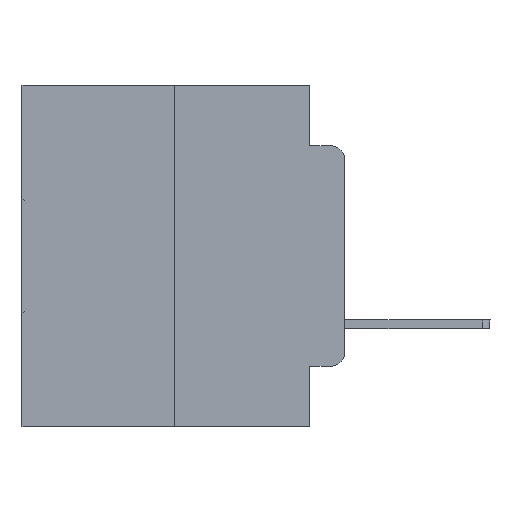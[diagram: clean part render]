
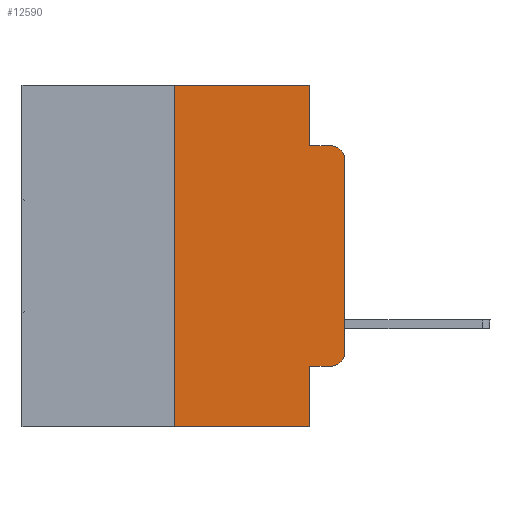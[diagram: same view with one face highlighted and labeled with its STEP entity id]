
A CAD part, left-side view. The second image highlights one B-rep face of the part: STEP entity #12590.
In plain terms, the highlighted planar face has unit normal (-1, 0, 0).
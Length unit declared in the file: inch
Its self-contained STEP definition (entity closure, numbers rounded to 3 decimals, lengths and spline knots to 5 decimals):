
#185 = DIRECTION ( 'NONE',  ( 0., -1., 0. ) ) ;
#440 = DIRECTION ( 'NONE',  ( 0., 0., -1. ) ) ;
#612 = CARTESIAN_POINT ( 'NONE',  ( 0., 0.051, -0.4115 ) ) ;
#1072 = VERTEX_POINT ( 'NONE', #17011 ) ;
#1355 = DIRECTION ( 'NONE',  ( 0., 0., 1. ) ) ;
#2196 = ORIENTED_EDGE ( 'NONE', *, *, #22453, .T. ) ;
#3520 = EDGE_CURVE ( 'NONE', #7182, #22280, #6328, .T. ) ;
#4024 = VECTOR ( 'NONE', #1355, 39.37008 ) ;
#4869 = VECTOR ( 'NONE', #11250, 39.37008 ) ;
#4883 = DIRECTION ( 'NONE',  ( 0., -1., 0. ) ) ;
#5035 = LINE ( 'NONE', #18570, #28274 ) ;
#5258 = LINE ( 'NONE', #19544, #15600 ) ;
#5340 = CARTESIAN_POINT ( 'NONE',  ( 0., 0.473, 0. ) ) ;
#5604 = CARTESIAN_POINT ( 'NONE',  ( 0., 0., 0. ) ) ;
#5632 = EDGE_CURVE ( 'NONE', #8315, #7182, #21976, .T. ) ;
#5678 = VECTOR ( 'NONE', #4883, 39.37008 ) ;
#5744 = VERTEX_POINT ( 'NONE', #24520 ) ;
#5757 = CARTESIAN_POINT ( 'NONE',  ( 0., 0.25, -0.5 ) ) ;
#5872 = AXIS2_PLACEMENT_3D ( 'NONE', #24093, #16868, #440 ) ;
#6207 = CARTESIAN_POINT ( 'NONE',  ( 0., 0.02, -0.3915 ) ) ;
#6328 = CIRCLE ( 'NONE', #5872, 0.02 ) ;
#7182 = VERTEX_POINT ( 'NONE', #18232 ) ;
#7201 = DIRECTION ( 'NONE',  ( 0., 0., -1. ) ) ;
#7538 = ORIENTED_EDGE ( 'NONE', *, *, #7728, .F. ) ;
#7728 = EDGE_CURVE ( 'NONE', #12987, #22280, #19800, .T. ) ;
#7964 = ORIENTED_EDGE ( 'NONE', *, *, #8859, .T. ) ;
#8315 = VERTEX_POINT ( 'NONE', #22614 ) ;
#8859 = EDGE_CURVE ( 'NONE', #1072, #8315, #14853, .T. ) ;
#9841 = EDGE_LOOP ( 'NONE', ( #21827, #12193, #7538, #10385, #12399, #19525, #2196, #14261, #29173, #7964 ) ) ;
#10385 = ORIENTED_EDGE ( 'NONE', *, *, #12627, .F. ) ;
#10553 = LINE ( 'NONE', #12821, #22631 ) ;
#11125 = CARTESIAN_POINT ( 'NONE',  ( 0., 0.051, 0. ) ) ;
#11250 = DIRECTION ( 'NONE',  ( 0., 0., -1. ) ) ;
#12193 = ORIENTED_EDGE ( 'NONE', *, *, #3520, .T. ) ;
#12399 = ORIENTED_EDGE ( 'NONE', *, *, #22517, .F. ) ;
#12590 = ADVANCED_FACE ( 'NONE', ( #26623 ), #12950, .F. ) ;
#12627 = EDGE_CURVE ( 'NONE', #15588, #12987, #29612, .T. ) ;
#12821 = CARTESIAN_POINT ( 'NONE',  ( 0., 0.051, 0. ) ) ;
#12950 = PLANE ( 'NONE',  #23628 ) ;
#12987 = VERTEX_POINT ( 'NONE', #13052 ) ;
#13052 = CARTESIAN_POINT ( 'NONE',  ( 0., 0.051, -0.0885 ) ) ;
#14261 = ORIENTED_EDGE ( 'NONE', *, *, #25723, .F. ) ;
#14439 = VERTEX_POINT ( 'NONE', #21592 ) ;
#14853 = CIRCLE ( 'NONE', #25391, 0.02 ) ;
#15588 = VERTEX_POINT ( 'NONE', #11125 ) ;
#15600 = VECTOR ( 'NONE', #26472, 39.37008 ) ;
#15680 = DIRECTION ( 'NONE',  ( 0., -1., 0. ) ) ;
#16063 = CARTESIAN_POINT ( 'NONE',  ( 0., 0.051, 0. ) ) ;
#16421 = EDGE_CURVE ( 'NONE', #22913, #1072, #20343, .T. ) ;
#16868 = DIRECTION ( 'NONE',  ( -1., 0., 0. ) ) ;
#17011 = CARTESIAN_POINT ( 'NONE',  ( 0., 0.02, -0.4115 ) ) ;
#17404 = DIRECTION ( 'NONE',  ( 0., -1., 0. ) ) ;
#17466 = DIRECTION ( 'NONE',  ( 0., 0., -1. ) ) ;
#17585 = CARTESIAN_POINT ( 'NONE',  ( 0., 0.473, 0. ) ) ;
#18105 = EDGE_CURVE ( 'NONE', #23099, #14439, #5258, .T. ) ;
#18232 = CARTESIAN_POINT ( 'NONE',  ( 0., 0., -0.1085 ) ) ;
#18570 = CARTESIAN_POINT ( 'NONE',  ( 0., 0.473, -0.5 ) ) ;
#19525 = ORIENTED_EDGE ( 'NONE', *, *, #18105, .F. ) ;
#19544 = CARTESIAN_POINT ( 'NONE',  ( 0., 0.25, 0. ) ) ;
#19800 = LINE ( 'NONE', #24177, #20542 ) ;
#20343 = LINE ( 'NONE', #22744, #21314 ) ;
#20542 = VECTOR ( 'NONE', #17404, 39.37008 ) ;
#20821 = LINE ( 'NONE', #5340, #5678 ) ;
#21314 = VECTOR ( 'NONE', #15680, 39.37008 ) ;
#21592 = CARTESIAN_POINT ( 'NONE',  ( 0., 0.25, 0. ) ) ;
#21827 = ORIENTED_EDGE ( 'NONE', *, *, #5632, .T. ) ;
#21976 = LINE ( 'NONE', #5604, #4024 ) ;
#22102 = DIRECTION ( 'NONE',  ( 1., 0., 0. ) ) ;
#22280 = VERTEX_POINT ( 'NONE', #28399 ) ;
#22396 = DIRECTION ( 'NONE',  ( 0., 0., -1. ) ) ;
#22453 = EDGE_CURVE ( 'NONE', #23099, #5744, #5035, .T. ) ;
#22517 = EDGE_CURVE ( 'NONE', #14439, #15588, #20821, .T. ) ;
#22614 = CARTESIAN_POINT ( 'NONE',  ( 0., 0., -0.3915 ) ) ;
#22631 = VECTOR ( 'NONE', #17466, 39.37008 ) ;
#22744 = CARTESIAN_POINT ( 'NONE',  ( 0., 0.051, -0.4115 ) ) ;
#22913 = VERTEX_POINT ( 'NONE', #612 ) ;
#23099 = VERTEX_POINT ( 'NONE', #5757 ) ;
#23628 = AXIS2_PLACEMENT_3D ( 'NONE', #17585, #22102, #22396 ) ;
#24093 = CARTESIAN_POINT ( 'NONE',  ( 0., 0.02, -0.1085 ) ) ;
#24177 = CARTESIAN_POINT ( 'NONE',  ( 0., 0.051, -0.0885 ) ) ;
#24520 = CARTESIAN_POINT ( 'NONE',  ( 0., 0.051, -0.5 ) ) ;
#25391 = AXIS2_PLACEMENT_3D ( 'NONE', #6207, #29083, #7201 ) ;
#25723 = EDGE_CURVE ( 'NONE', #22913, #5744, #10553, .T. ) ;
#26472 = DIRECTION ( 'NONE',  ( 0., 0., 1. ) ) ;
#26623 = FACE_OUTER_BOUND ( 'NONE', #9841, .T. ) ;
#28274 = VECTOR ( 'NONE', #185, 39.37008 ) ;
#28399 = CARTESIAN_POINT ( 'NONE',  ( 0., 0.02, -0.0885 ) ) ;
#29083 = DIRECTION ( 'NONE',  ( -1., 0., 0. ) ) ;
#29173 = ORIENTED_EDGE ( 'NONE', *, *, #16421, .T. ) ;
#29612 = LINE ( 'NONE', #16063, #4869 ) ;
